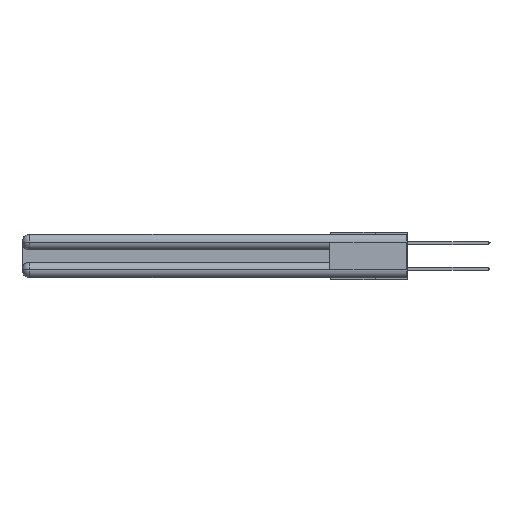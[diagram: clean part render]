
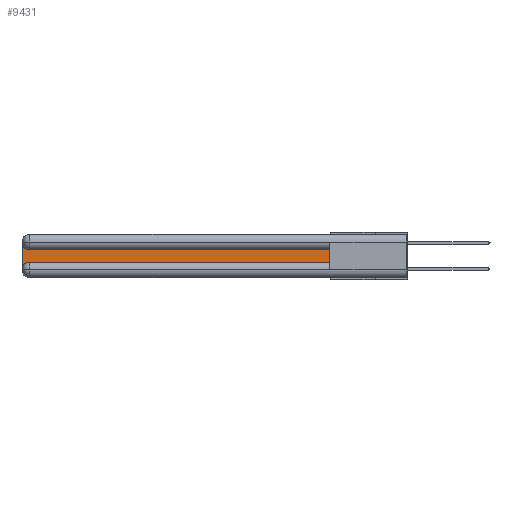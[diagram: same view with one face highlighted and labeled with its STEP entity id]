
A CAD part, left-side view. The second image highlights one B-rep face of the part: STEP entity #9431.
In plain terms, the highlighted planar face has unit normal (-1, 0, 0).
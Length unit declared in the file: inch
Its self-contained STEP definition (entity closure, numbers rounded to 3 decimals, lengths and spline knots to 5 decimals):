
#220 = ORIENTED_EDGE ( 'NONE', *, *, #21994, .T. ) ;
#918 = EDGE_CURVE ( 'NONE', #19675, #15290, #25902, .T. ) ;
#1954 = DIRECTION ( 'NONE',  ( 0., 0., -1. ) ) ;
#3330 = VECTOR ( 'NONE', #26988, 39.37008 ) ;
#3432 = CARTESIAN_POINT ( 'NONE',  ( 0.075, 2.94, -0.2775 ) ) ;
#4839 = CARTESIAN_POINT ( 'NONE',  ( 0.075, 3., -0.2775 ) ) ;
#5387 = FACE_OUTER_BOUND ( 'NONE', #7603, .T. ) ;
#5396 = DIRECTION ( 'NONE',  ( 0., 0., -1. ) ) ;
#5622 = CARTESIAN_POINT ( 'NONE',  ( 0.075, 2.94, -0.2175 ) ) ;
#5691 = CARTESIAN_POINT ( 'NONE',  ( 0.075, 2.94, -0.0625 ) ) ;
#6060 = ORIENTED_EDGE ( 'NONE', *, *, #918, .T. ) ;
#7454 = CARTESIAN_POINT ( 'NONE',  ( 0.075, 0.6, -0.2175 ) ) ;
#7603 = EDGE_LOOP ( 'NONE', ( #8271, #6060, #22742, #15343, #220, #7834 ) ) ;
#7650 = VECTOR ( 'NONE', #11831, 39.37008 ) ;
#7834 = ORIENTED_EDGE ( 'NONE', *, *, #10046, .T. ) ;
#8005 = CIRCLE ( 'NONE', #28370, 0.06 ) ;
#8271 = ORIENTED_EDGE ( 'NONE', *, *, #17928, .T. ) ;
#8383 = LINE ( 'NONE', #7454, #7650 ) ;
#9431 = ADVANCED_FACE ( 'NONE', ( #5387 ), #27417, .F. ) ;
#9750 = CARTESIAN_POINT ( 'NONE',  ( 0.075, 3., -0.0625 ) ) ;
#10046 = EDGE_CURVE ( 'NONE', #14628, #26250, #11189, .T. ) ;
#11189 = LINE ( 'NONE', #22074, #28198 ) ;
#11831 = DIRECTION ( 'NONE',  ( 0., -1., 0. ) ) ;
#13735 = VERTEX_POINT ( 'NONE', #5622 ) ;
#14076 = VECTOR ( 'NONE', #22239, 39.37008 ) ;
#14628 = VERTEX_POINT ( 'NONE', #29163 ) ;
#14630 = AXIS2_PLACEMENT_3D ( 'NONE', #29768, #15892, #1954 ) ;
#15074 = CARTESIAN_POINT ( 'NONE',  ( 0.075, 3., -0.2175 ) ) ;
#15122 = DIRECTION ( 'NONE',  ( 0., 0., 1. ) ) ;
#15290 = VERTEX_POINT ( 'NONE', #9750 ) ;
#15343 = ORIENTED_EDGE ( 'NONE', *, *, #22208, .T. ) ;
#15474 = CARTESIAN_POINT ( 'NONE',  ( 0.075, 0.6, -0.1225 ) ) ;
#15892 = DIRECTION ( 'NONE',  ( 1., 0., 0. ) ) ;
#17928 = EDGE_CURVE ( 'NONE', #26250, #19675, #26905, .T. ) ;
#19412 = AXIS2_PLACEMENT_3D ( 'NONE', #5691, #28797, #5396 ) ;
#19675 = VERTEX_POINT ( 'NONE', #26798 ) ;
#19692 = DIRECTION ( 'NONE',  ( 1., 0., 0. ) ) ;
#19913 = CARTESIAN_POINT ( 'NONE',  ( 0.075, 0.6, -0.1225 ) ) ;
#21633 = LINE ( 'NONE', #15074, #14076 ) ;
#21994 = EDGE_CURVE ( 'NONE', #13735, #14628, #8383, .T. ) ;
#22074 = CARTESIAN_POINT ( 'NONE',  ( 0.075, 0.6, -0.2175 ) ) ;
#22208 = EDGE_CURVE ( 'NONE', #27439, #13735, #8005, .T. ) ;
#22239 = DIRECTION ( 'NONE',  ( 0., 0., -1. ) ) ;
#22742 = ORIENTED_EDGE ( 'NONE', *, *, #23937, .T. ) ;
#23937 = EDGE_CURVE ( 'NONE', #15290, #27439, #21633, .T. ) ;
#24702 = DIRECTION ( 'NONE',  ( 0., 0., -1. ) ) ;
#25902 = CIRCLE ( 'NONE', #19412, 0.06 ) ;
#26250 = VERTEX_POINT ( 'NONE', #19913 ) ;
#26798 = CARTESIAN_POINT ( 'NONE',  ( 0.075, 2.94, -0.1225 ) ) ;
#26905 = LINE ( 'NONE', #15474, #3330 ) ;
#26988 = DIRECTION ( 'NONE',  ( 0., 1., 0. ) ) ;
#27417 = PLANE ( 'NONE',  #14630 ) ;
#27439 = VERTEX_POINT ( 'NONE', #4839 ) ;
#28198 = VECTOR ( 'NONE', #15122, 39.37008 ) ;
#28370 = AXIS2_PLACEMENT_3D ( 'NONE', #3432, #19692, #24702 ) ;
#28797 = DIRECTION ( 'NONE',  ( 1., 0., 0. ) ) ;
#29163 = CARTESIAN_POINT ( 'NONE',  ( 0.075, 0.6, -0.2175 ) ) ;
#29768 = CARTESIAN_POINT ( 'NONE',  ( 0.075, 3., -0.1225 ) ) ;
